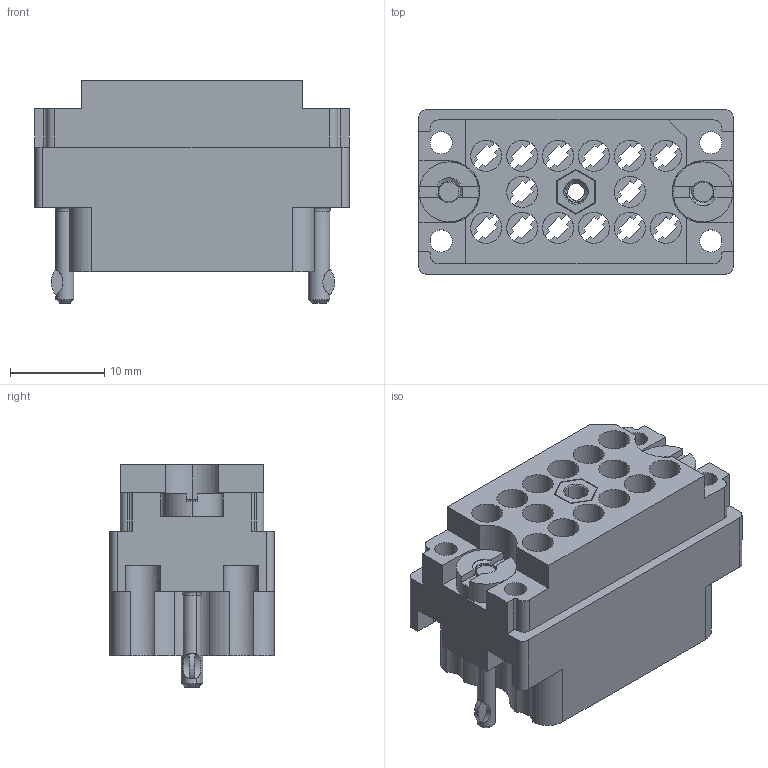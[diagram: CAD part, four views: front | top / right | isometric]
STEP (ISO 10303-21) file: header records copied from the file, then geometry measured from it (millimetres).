
FILE_DESCRIPTION (( 'STEP AP203' ), '1' );
FILE_NAME ('519-014-000-302.STEP', '2020-03-11T15:48:57', ( '' ), ( '' ), 'SwSTEP 2.0', 'SolidWorks 2016', '' );
FILE_SCHEMA (( 'CONFIG_CONTROL_DESIGN' ));
Length unit declared in the file: inch
Products named in the file (6): 516-222-020-102_015; 516-252-025-100_516-252-025-100; 519 Plug Insulator_014; 519-014-000-302; 516-222-020-102_014; 516-252-021-102_014
Assembly tree (6 placements, depth 2):
  519-014-000-302
    519 Plug Insulator_014
    516-252-025-100_516-252-025-100
    516-252-021-102_014  x2
    516-222-020-102_014
    516-222-020-102_015
Bounding box: 33.32 x 17.42 x 23.6 mm (x, y, z)
Volume: 5387.6 mm3; surface area: 7061.5 mm2
Topology: 6 solids, 6 shells, 740 faces, 2079 edges, 1366 vertices
Faces by surface type: plane 382, cylinder 266, cone 49, bspline 39, torus 4
Entity records: 30334 total; most frequent: CARTESIAN_POINT 11468, ORIENTED_EDGE 3978, DIRECTION 3673, EDGE_CURVE 1989, VERTEX_POINT 1306, AXIS2_PLACEMENT_3D 1232, LINE 1209, VECTOR 1209
